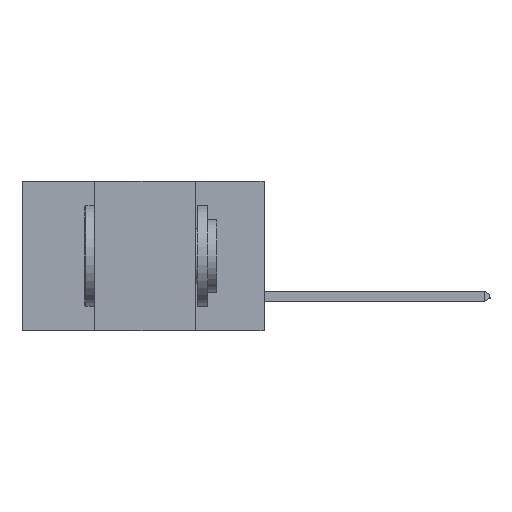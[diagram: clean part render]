
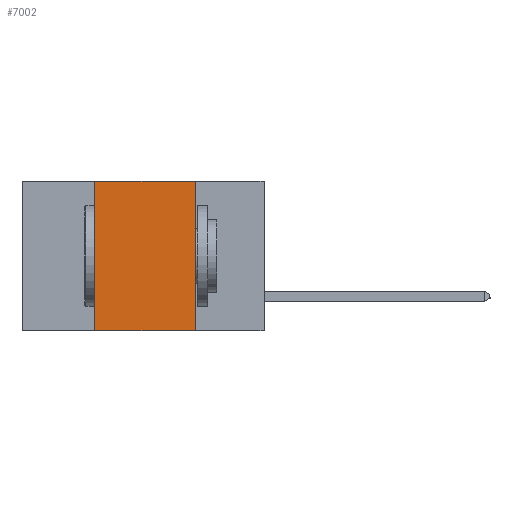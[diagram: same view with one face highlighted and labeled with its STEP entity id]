
A CAD part, left-side view. The second image highlights one B-rep face of the part: STEP entity #7002.
In plain terms, the highlighted planar face has unit normal (-1, 0, 0).
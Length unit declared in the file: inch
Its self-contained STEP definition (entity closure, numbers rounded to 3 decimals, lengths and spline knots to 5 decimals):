
#851 = ORIENTED_EDGE ( 'NONE', *, *, #2774, .T. ) ;
#998 = CARTESIAN_POINT ( 'NONE',  ( 0., 0.6, 0. ) ) ;
#1394 = CARTESIAN_POINT ( 'NONE',  ( 0., 0.17, 0. ) ) ;
#1491 = AXIS2_PLACEMENT_3D ( 'NONE', #1527, #12344, #3086 ) ;
#1523 = DIRECTION ( 'NONE',  ( 0., 0., 1. ) ) ;
#1527 = CARTESIAN_POINT ( 'NONE',  ( 0., 0.6, 0. ) ) ;
#1889 = ORIENTED_EDGE ( 'NONE', *, *, #3332, .F. ) ;
#2610 = CARTESIAN_POINT ( 'NONE',  ( 0., 0.42, 0. ) ) ;
#2774 = EDGE_CURVE ( 'NONE', #16170, #10448, #17750, .T. ) ;
#3086 = DIRECTION ( 'NONE',  ( 0., 0., -1. ) ) ;
#3199 = FACE_OUTER_BOUND ( 'NONE', #7718, .T. ) ;
#3332 = EDGE_CURVE ( 'NONE', #19754, #11553, #16109, .T. ) ;
#4189 = LINE ( 'NONE', #1394, #12387 ) ;
#4658 = VECTOR ( 'NONE', #1523, 39.37008 ) ;
#4883 = EDGE_CURVE ( 'NONE', #16170, #19754, #16960, .T. ) ;
#4985 = ORIENTED_EDGE ( 'NONE', *, *, #6960, .F. ) ;
#5994 = VECTOR ( 'NONE', #19351, 39.37008 ) ;
#6960 = EDGE_CURVE ( 'NONE', #11553, #10448, #4189, .T. ) ;
#7002 = ADVANCED_FACE ( 'NONE', ( #3199 ), #10844, .F. ) ;
#7718 = EDGE_LOOP ( 'NONE', ( #4985, #1889, #8135, #851 ) ) ;
#8135 = ORIENTED_EDGE ( 'NONE', *, *, #4883, .F. ) ;
#10448 = VERTEX_POINT ( 'NONE', #19570 ) ;
#10537 = CARTESIAN_POINT ( 'NONE',  ( 0., 0.17, 0. ) ) ;
#10844 = PLANE ( 'NONE',  #1491 ) ;
#11151 = CARTESIAN_POINT ( 'NONE',  ( 0., 0.42, 0. ) ) ;
#11553 = VERTEX_POINT ( 'NONE', #10537 ) ;
#11673 = DIRECTION ( 'NONE',  ( 0., -1., 0. ) ) ;
#12344 = DIRECTION ( 'NONE',  ( 1., 0., 0. ) ) ;
#12387 = VECTOR ( 'NONE', #16826, 39.37008 ) ;
#15176 = CARTESIAN_POINT ( 'NONE',  ( 0., 0.42, -0.37 ) ) ;
#16109 = LINE ( 'NONE', #998, #19493 ) ;
#16170 = VERTEX_POINT ( 'NONE', #15176 ) ;
#16826 = DIRECTION ( 'NONE',  ( 0., 0., -1. ) ) ;
#16960 = LINE ( 'NONE', #2610, #4658 ) ;
#17750 = LINE ( 'NONE', #19392, #5994 ) ;
#19351 = DIRECTION ( 'NONE',  ( 0., -1., 0. ) ) ;
#19392 = CARTESIAN_POINT ( 'NONE',  ( 0., 0.6, -0.37 ) ) ;
#19493 = VECTOR ( 'NONE', #11673, 39.37008 ) ;
#19570 = CARTESIAN_POINT ( 'NONE',  ( 0., 0.17, -0.37 ) ) ;
#19754 = VERTEX_POINT ( 'NONE', #11151 ) ;
